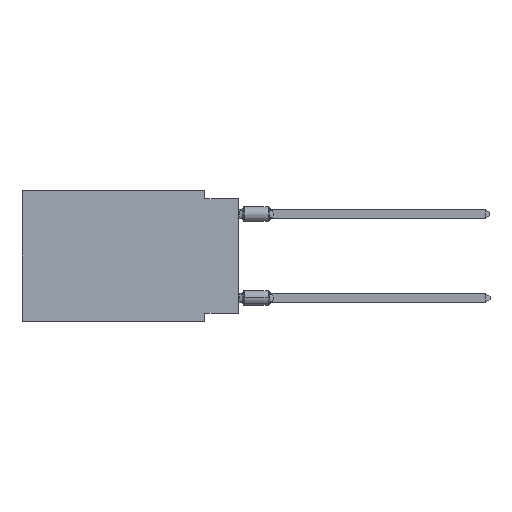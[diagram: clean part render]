
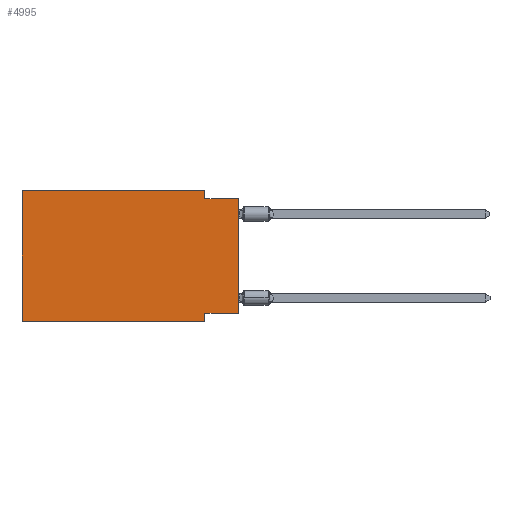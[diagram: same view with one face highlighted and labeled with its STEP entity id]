
A CAD part, left-side view. The second image highlights one B-rep face of the part: STEP entity #4995.
In plain terms, the highlighted planar face has unit normal (-1, 0, 0).
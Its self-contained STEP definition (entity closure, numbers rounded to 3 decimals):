
#45 = CARTESIAN_POINT ( 'NONE',  ( 0., 16.383, 0. ) ) ;
#773 = EDGE_CURVE ( 'NONE', #10566, #20608, #23595, .T. ) ;
#2039 = EDGE_CURVE ( 'NONE', #14540, #10566, #13924, .T. ) ;
#3103 = CARTESIAN_POINT ( 'NONE',  ( 0., 2.54, -9.271 ) ) ;
#3141 = LINE ( 'NONE', #26075, #24683 ) ;
#3495 = CARTESIAN_POINT ( 'NONE',  ( 0., 16.383, -9.906 ) ) ;
#4235 = VECTOR ( 'NONE', #23146, 1000. ) ;
#4254 = EDGE_CURVE ( 'NONE', #4896, #11675, #7051, .T. ) ;
#4769 = CARTESIAN_POINT ( 'NONE',  ( 0., 16.383, 0. ) ) ;
#4896 = VERTEX_POINT ( 'NONE', #21016 ) ;
#4995 = ADVANCED_FACE ( 'NONE', ( #25491 ), #6823, .F. ) ;
#5073 = AXIS2_PLACEMENT_3D ( 'NONE', #4769, #13125, #21423 ) ;
#5725 = EDGE_CURVE ( 'NONE', #23826, #7128, #3141, .T. ) ;
#6213 = VECTOR ( 'NONE', #8373, 1000. ) ;
#6823 = PLANE ( 'NONE',  #5073 ) ;
#7051 = LINE ( 'NONE', #16280, #9823 ) ;
#7128 = VERTEX_POINT ( 'NONE', #13465 ) ;
#7263 = DIRECTION ( 'NONE',  ( 0., 0., 1. ) ) ;
#7768 = DIRECTION ( 'NONE',  ( 0., 0., -1. ) ) ;
#7922 = DIRECTION ( 'NONE',  ( 0., -1., 0. ) ) ;
#8373 = DIRECTION ( 'NONE',  ( 0., -1., 0. ) ) ;
#9702 = DIRECTION ( 'NONE',  ( 0., 0., 1. ) ) ;
#9813 = CARTESIAN_POINT ( 'NONE',  ( 0., 2.54, 0. ) ) ;
#9823 = VECTOR ( 'NONE', #24570, 1000. ) ;
#10566 = VERTEX_POINT ( 'NONE', #12499 ) ;
#11333 = DIRECTION ( 'NONE',  ( 0., -1., 0. ) ) ;
#11365 = ORIENTED_EDGE ( 'NONE', *, *, #773, .F. ) ;
#11494 = CARTESIAN_POINT ( 'NONE',  ( 0., 0., 0. ) ) ;
#11675 = VERTEX_POINT ( 'NONE', #3103 ) ;
#11785 = LINE ( 'NONE', #11494, #13032 ) ;
#11939 = VECTOR ( 'NONE', #7922, 1000. ) ;
#12107 = ORIENTED_EDGE ( 'NONE', *, *, #2039, .F. ) ;
#12499 = CARTESIAN_POINT ( 'NONE',  ( 0., 2.54, -0.635 ) ) ;
#12645 = VECTOR ( 'NONE', #7768, 1000. ) ;
#13032 = VECTOR ( 'NONE', #9702, 1000. ) ;
#13125 = DIRECTION ( 'NONE',  ( 1., 0., 0. ) ) ;
#13464 = VECTOR ( 'NONE', #11333, 1000. ) ;
#13465 = CARTESIAN_POINT ( 'NONE',  ( 0., 16.383, 0. ) ) ;
#13924 = LINE ( 'NONE', #14190, #12645 ) ;
#14059 = EDGE_CURVE ( 'NONE', #4896, #20608, #11785, .T. ) ;
#14190 = CARTESIAN_POINT ( 'NONE',  ( 0., 2.54, 0. ) ) ;
#14540 = VERTEX_POINT ( 'NONE', #9813 ) ;
#14795 = VERTEX_POINT ( 'NONE', #21282 ) ;
#14853 = LINE ( 'NONE', #16881, #4235 ) ;
#15709 = CARTESIAN_POINT ( 'NONE',  ( 0., 0., -0.635 ) ) ;
#16280 = CARTESIAN_POINT ( 'NONE',  ( 0., 0., -9.271 ) ) ;
#16625 = ORIENTED_EDGE ( 'NONE', *, *, #4254, .F. ) ;
#16740 = ORIENTED_EDGE ( 'NONE', *, *, #24494, .F. ) ;
#16881 = CARTESIAN_POINT ( 'NONE',  ( 0., 2.54, -9.906 ) ) ;
#18409 = LINE ( 'NONE', #26720, #11939 ) ;
#18753 = LINE ( 'NONE', #45, #6213 ) ;
#20037 = ORIENTED_EDGE ( 'NONE', *, *, #5725, .F. ) ;
#20453 = ORIENTED_EDGE ( 'NONE', *, *, #26531, .T. ) ;
#20608 = VERTEX_POINT ( 'NONE', #22365 ) ;
#21016 = CARTESIAN_POINT ( 'NONE',  ( 0., 0., -9.271 ) ) ;
#21262 = ORIENTED_EDGE ( 'NONE', *, *, #14059, .T. ) ;
#21282 = CARTESIAN_POINT ( 'NONE',  ( 0., 2.54, -9.906 ) ) ;
#21423 = DIRECTION ( 'NONE',  ( 0., 0., -1. ) ) ;
#22365 = CARTESIAN_POINT ( 'NONE',  ( 0., 0., -0.635 ) ) ;
#22440 = EDGE_CURVE ( 'NONE', #11675, #14795, #14853, .T. ) ;
#23146 = DIRECTION ( 'NONE',  ( 0., 0., -1. ) ) ;
#23503 = ORIENTED_EDGE ( 'NONE', *, *, #22440, .F. ) ;
#23595 = LINE ( 'NONE', #15709, #13464 ) ;
#23826 = VERTEX_POINT ( 'NONE', #3495 ) ;
#24494 = EDGE_CURVE ( 'NONE', #7128, #14540, #18753, .T. ) ;
#24570 = DIRECTION ( 'NONE',  ( 0., 1., 0. ) ) ;
#24683 = VECTOR ( 'NONE', #7263, 1000. ) ;
#25006 = EDGE_LOOP ( 'NONE', ( #21262, #11365, #12107, #16740, #20037, #20453, #23503, #16625 ) ) ;
#25491 = FACE_OUTER_BOUND ( 'NONE', #25006, .T. ) ;
#26075 = CARTESIAN_POINT ( 'NONE',  ( 0., 16.383, 0. ) ) ;
#26531 = EDGE_CURVE ( 'NONE', #23826, #14795, #18409, .T. ) ;
#26720 = CARTESIAN_POINT ( 'NONE',  ( 0., 16.383, -9.906 ) ) ;
